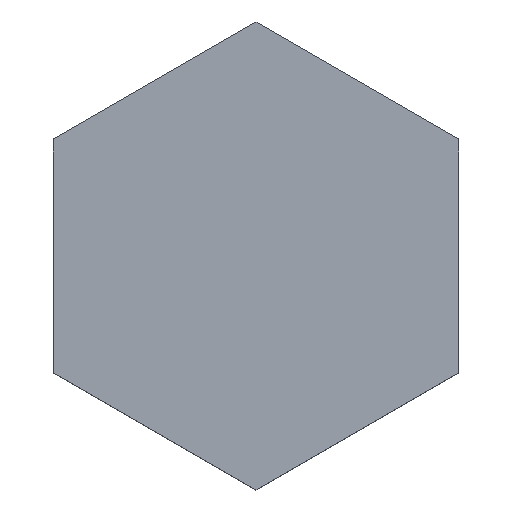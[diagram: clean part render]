
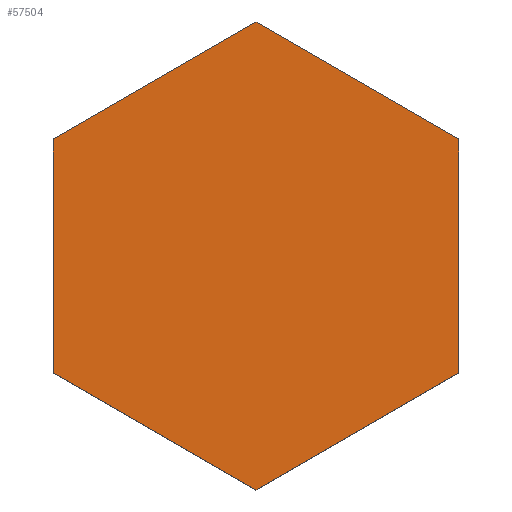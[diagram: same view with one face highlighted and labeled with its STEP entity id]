
A CAD part, top view. The second image highlights one B-rep face of the part: STEP entity #57504.
In plain terms, the highlighted planar face has unit normal (0, 0, 1).
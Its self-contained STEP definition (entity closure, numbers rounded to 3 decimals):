
#56753 = PLANE('',#56754);
#56754 = AXIS2_PLACEMENT_3D('',#56755,#56756,#56757);
#56755 = CARTESIAN_POINT('',(0.,19.05,-151.968));
#56756 = DIRECTION('',(-0.5,0.866,0.));
#56757 = DIRECTION('',(-0.866,-0.5,0.));
#56781 = PLANE('',#56782);
#56782 = AXIS2_PLACEMENT_3D('',#56783,#56784,#56785);
#56783 = CARTESIAN_POINT('',(16.498,9.525,-151.968));
#56784 = DIRECTION('',(0.5,0.866,0.));
#56785 = DIRECTION('',(-0.866,0.5,0.));
#56809 = PLANE('',#56810);
#56810 = AXIS2_PLACEMENT_3D('',#56811,#56812,#56813);
#56811 = CARTESIAN_POINT('',(16.498,-9.525,-151.968));
#56812 = DIRECTION('',(1.,0.,0.));
#56813 = DIRECTION('',(0.,1.,0.));
#56837 = PLANE('',#56838);
#56838 = AXIS2_PLACEMENT_3D('',#56839,#56840,#56841);
#56839 = CARTESIAN_POINT('',(0.,-19.05,-151.968));
#56840 = DIRECTION('',(0.5,-0.866,0.));
#56841 = DIRECTION('',(0.866,0.5,0.));
#56865 = PLANE('',#56866);
#56866 = AXIS2_PLACEMENT_3D('',#56867,#56868,#56869);
#56867 = CARTESIAN_POINT('',(-16.498,-9.525,-151.968));
#56868 = DIRECTION('',(-0.5,-0.866,0.));
#56869 = DIRECTION('',(0.866,-0.5,0.));
#56891 = PLANE('',#56892);
#56892 = AXIS2_PLACEMENT_3D('',#56893,#56894,#56895);
#56893 = CARTESIAN_POINT('',(-16.498,9.525,-151.968));
#56894 = DIRECTION('',(-1.,0.,0.));
#56895 = DIRECTION('',(0.,-1.,0.));
#57099 = VERTEX_POINT('',#57100);
#57100 = CARTESIAN_POINT('',(-16.498,9.525,-151.968));
#57121 = EDGE_CURVE('',#57122,#57099,#57124,.T.);
#57122 = VERTEX_POINT('',#57123);
#57123 = CARTESIAN_POINT('',(0.,19.05,-151.968));
#57124 = SURFACE_CURVE('',#57125,(#57129,#57136),.PCURVE_S1.);
#57125 = LINE('',#57126,#57127);
#57126 = CARTESIAN_POINT('',(0.,19.05,-151.968));
#57127 = VECTOR('',#57128,1.);
#57128 = DIRECTION('',(-0.866,-0.5,0.));
#57129 = PCURVE('',#56753,#57130);
#57130 = DEFINITIONAL_REPRESENTATION('',(#57131),#57135);
#57131 = LINE('',#57132,#57133);
#57132 = CARTESIAN_POINT('',(0.,0.));
#57133 = VECTOR('',#57134,1.);
#57134 = DIRECTION('',(1.,0.));
#57135 = ( GEOMETRIC_REPRESENTATION_CONTEXT(2) 
PARAMETRIC_REPRESENTATION_CONTEXT() REPRESENTATION_CONTEXT('2D SPACE',''
  ) );
#57136 = PCURVE('',#57137,#57142);
#57137 = PLANE('',#57138);
#57138 = AXIS2_PLACEMENT_3D('',#57139,#57140,#57141);
#57139 = CARTESIAN_POINT('',(-7.278,22.416,-151.968));
#57140 = DIRECTION('',(0.,0.,-1.));
#57141 = DIRECTION('',(-1.,0.,0.));
#57142 = DEFINITIONAL_REPRESENTATION('',(#57143),#57147);
#57143 = LINE('',#57144,#57145);
#57144 = CARTESIAN_POINT('',(-7.278,-3.366));
#57145 = VECTOR('',#57146,1.);
#57146 = DIRECTION('',(0.866,-0.5));
#57147 = ( GEOMETRIC_REPRESENTATION_CONTEXT(2) 
PARAMETRIC_REPRESENTATION_CONTEXT() REPRESENTATION_CONTEXT('2D SPACE',''
  ) );
#57175 = EDGE_CURVE('',#57176,#57122,#57178,.T.);
#57176 = VERTEX_POINT('',#57177);
#57177 = CARTESIAN_POINT('',(16.498,9.525,-151.968));
#57178 = SURFACE_CURVE('',#57179,(#57183,#57190),.PCURVE_S1.);
#57179 = LINE('',#57180,#57181);
#57180 = CARTESIAN_POINT('',(16.498,9.525,-151.968));
#57181 = VECTOR('',#57182,1.);
#57182 = DIRECTION('',(-0.866,0.5,0.));
#57183 = PCURVE('',#56781,#57184);
#57184 = DEFINITIONAL_REPRESENTATION('',(#57185),#57189);
#57185 = LINE('',#57186,#57187);
#57186 = CARTESIAN_POINT('',(0.,0.));
#57187 = VECTOR('',#57188,1.);
#57188 = DIRECTION('',(1.,0.));
#57189 = ( GEOMETRIC_REPRESENTATION_CONTEXT(2) 
PARAMETRIC_REPRESENTATION_CONTEXT() REPRESENTATION_CONTEXT('2D SPACE',''
  ) );
#57190 = PCURVE('',#57137,#57191);
#57191 = DEFINITIONAL_REPRESENTATION('',(#57192),#57196);
#57192 = LINE('',#57193,#57194);
#57193 = CARTESIAN_POINT('',(-23.776,-12.891));
#57194 = VECTOR('',#57195,1.);
#57195 = DIRECTION('',(0.866,0.5));
#57196 = ( GEOMETRIC_REPRESENTATION_CONTEXT(2) 
PARAMETRIC_REPRESENTATION_CONTEXT() REPRESENTATION_CONTEXT('2D SPACE',''
  ) );
#57224 = EDGE_CURVE('',#57225,#57176,#57227,.T.);
#57225 = VERTEX_POINT('',#57226);
#57226 = CARTESIAN_POINT('',(16.498,-9.525,-151.968));
#57227 = SURFACE_CURVE('',#57228,(#57232,#57239),.PCURVE_S1.);
#57228 = LINE('',#57229,#57230);
#57229 = CARTESIAN_POINT('',(16.498,-9.525,-151.968));
#57230 = VECTOR('',#57231,1.);
#57231 = DIRECTION('',(0.,1.,0.));
#57232 = PCURVE('',#56809,#57233);
#57233 = DEFINITIONAL_REPRESENTATION('',(#57234),#57238);
#57234 = LINE('',#57235,#57236);
#57235 = CARTESIAN_POINT('',(0.,0.));
#57236 = VECTOR('',#57237,1.);
#57237 = DIRECTION('',(1.,0.));
#57238 = ( GEOMETRIC_REPRESENTATION_CONTEXT(2) 
PARAMETRIC_REPRESENTATION_CONTEXT() REPRESENTATION_CONTEXT('2D SPACE',''
  ) );
#57239 = PCURVE('',#57137,#57240);
#57240 = DEFINITIONAL_REPRESENTATION('',(#57241),#57245);
#57241 = LINE('',#57242,#57243);
#57242 = CARTESIAN_POINT('',(-23.776,-31.941));
#57243 = VECTOR('',#57244,1.);
#57244 = DIRECTION('',(0.,1.));
#57245 = ( GEOMETRIC_REPRESENTATION_CONTEXT(2) 
PARAMETRIC_REPRESENTATION_CONTEXT() REPRESENTATION_CONTEXT('2D SPACE',''
  ) );
#57273 = EDGE_CURVE('',#57274,#57225,#57276,.T.);
#57274 = VERTEX_POINT('',#57275);
#57275 = CARTESIAN_POINT('',(0.,-19.05,-151.968));
#57276 = SURFACE_CURVE('',#57277,(#57281,#57288),.PCURVE_S1.);
#57277 = LINE('',#57278,#57279);
#57278 = CARTESIAN_POINT('',(0.,-19.05,-151.968));
#57279 = VECTOR('',#57280,1.);
#57280 = DIRECTION('',(0.866,0.5,0.));
#57281 = PCURVE('',#56837,#57282);
#57282 = DEFINITIONAL_REPRESENTATION('',(#57283),#57287);
#57283 = LINE('',#57284,#57285);
#57284 = CARTESIAN_POINT('',(0.,0.));
#57285 = VECTOR('',#57286,1.);
#57286 = DIRECTION('',(1.,0.));
#57287 = ( GEOMETRIC_REPRESENTATION_CONTEXT(2) 
PARAMETRIC_REPRESENTATION_CONTEXT() REPRESENTATION_CONTEXT('2D SPACE',''
  ) );
#57288 = PCURVE('',#57137,#57289);
#57289 = DEFINITIONAL_REPRESENTATION('',(#57290),#57294);
#57290 = LINE('',#57291,#57292);
#57291 = CARTESIAN_POINT('',(-7.278,-41.466));
#57292 = VECTOR('',#57293,1.);
#57293 = DIRECTION('',(-0.866,0.5));
#57294 = ( GEOMETRIC_REPRESENTATION_CONTEXT(2) 
PARAMETRIC_REPRESENTATION_CONTEXT() REPRESENTATION_CONTEXT('2D SPACE',''
  ) );
#57322 = EDGE_CURVE('',#57323,#57274,#57325,.T.);
#57323 = VERTEX_POINT('',#57324);
#57324 = CARTESIAN_POINT('',(-16.498,-9.525,-151.968));
#57325 = SURFACE_CURVE('',#57326,(#57330,#57337),.PCURVE_S1.);
#57326 = LINE('',#57327,#57328);
#57327 = CARTESIAN_POINT('',(-16.498,-9.525,-151.968));
#57328 = VECTOR('',#57329,1.);
#57329 = DIRECTION('',(0.866,-0.5,0.));
#57330 = PCURVE('',#56865,#57331);
#57331 = DEFINITIONAL_REPRESENTATION('',(#57332),#57336);
#57332 = LINE('',#57333,#57334);
#57333 = CARTESIAN_POINT('',(0.,0.));
#57334 = VECTOR('',#57335,1.);
#57335 = DIRECTION('',(1.,0.));
#57336 = ( GEOMETRIC_REPRESENTATION_CONTEXT(2) 
PARAMETRIC_REPRESENTATION_CONTEXT() REPRESENTATION_CONTEXT('2D SPACE',''
  ) );
#57337 = PCURVE('',#57137,#57338);
#57338 = DEFINITIONAL_REPRESENTATION('',(#57339),#57343);
#57339 = LINE('',#57340,#57341);
#57340 = CARTESIAN_POINT('',(9.219,-31.941));
#57341 = VECTOR('',#57342,1.);
#57342 = DIRECTION('',(-0.866,-0.5));
#57343 = ( GEOMETRIC_REPRESENTATION_CONTEXT(2) 
PARAMETRIC_REPRESENTATION_CONTEXT() REPRESENTATION_CONTEXT('2D SPACE',''
  ) );
#57371 = EDGE_CURVE('',#57099,#57323,#57372,.T.);
#57372 = SURFACE_CURVE('',#57373,(#57377,#57384),.PCURVE_S1.);
#57373 = LINE('',#57374,#57375);
#57374 = CARTESIAN_POINT('',(-16.498,9.525,-151.968));
#57375 = VECTOR('',#57376,1.);
#57376 = DIRECTION('',(0.,-1.,0.));
#57377 = PCURVE('',#56891,#57378);
#57378 = DEFINITIONAL_REPRESENTATION('',(#57379),#57383);
#57379 = LINE('',#57380,#57381);
#57380 = CARTESIAN_POINT('',(0.,0.));
#57381 = VECTOR('',#57382,1.);
#57382 = DIRECTION('',(1.,0.));
#57383 = ( GEOMETRIC_REPRESENTATION_CONTEXT(2) 
PARAMETRIC_REPRESENTATION_CONTEXT() REPRESENTATION_CONTEXT('2D SPACE',''
  ) );
#57384 = PCURVE('',#57137,#57385);
#57385 = DEFINITIONAL_REPRESENTATION('',(#57386),#57390);
#57386 = LINE('',#57387,#57388);
#57387 = CARTESIAN_POINT('',(9.219,-12.891));
#57388 = VECTOR('',#57389,1.);
#57389 = DIRECTION('',(0.,-1.));
#57390 = ( GEOMETRIC_REPRESENTATION_CONTEXT(2) 
PARAMETRIC_REPRESENTATION_CONTEXT() REPRESENTATION_CONTEXT('2D SPACE',''
  ) );
#57504 = ADVANCED_FACE('',(#57505),#57137,.F.);
#57505 = FACE_BOUND('',#57506,.T.);
#57506 = EDGE_LOOP('',(#57507,#57508,#57509,#57510,#57511,#57512));
#57507 = ORIENTED_EDGE('',*,*,#57322,.T.);
#57508 = ORIENTED_EDGE('',*,*,#57273,.T.);
#57509 = ORIENTED_EDGE('',*,*,#57224,.T.);
#57510 = ORIENTED_EDGE('',*,*,#57175,.T.);
#57511 = ORIENTED_EDGE('',*,*,#57121,.T.);
#57512 = ORIENTED_EDGE('',*,*,#57371,.T.);
